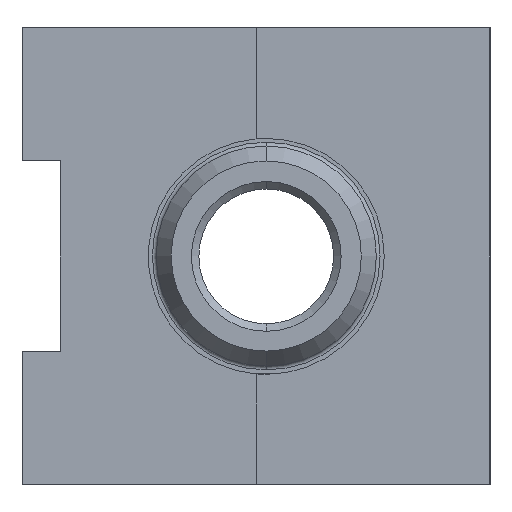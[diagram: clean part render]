
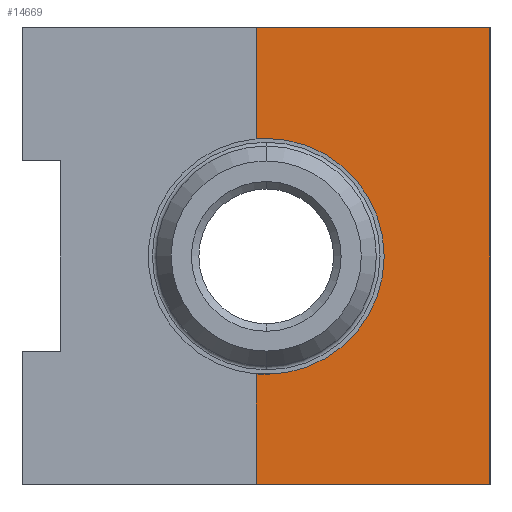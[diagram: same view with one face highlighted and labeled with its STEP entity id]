
A CAD part, left-side view. The second image highlights one B-rep face of the part: STEP entity #14669.
In plain terms, the highlighted face is planar.
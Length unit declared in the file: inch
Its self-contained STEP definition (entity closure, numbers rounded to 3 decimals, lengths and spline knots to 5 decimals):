
#445 = CARTESIAN_POINT ( 'NONE',  ( 1.2, -0.615, 0. ) ) ;
#660 = DIRECTION ( 'NONE',  ( 0., 1., 0. ) ) ;
#760 = DIRECTION ( 'NONE',  ( 1., 0., 0. ) ) ;
#808 = LINE ( 'NONE', #13899, #10339 ) ;
#1237 = VECTOR ( 'NONE', #19459, 39.37008 ) ;
#3102 = CARTESIAN_POINT ( 'NONE',  ( 0.29219, -0.615, 0. ) ) ;
#3241 = DIRECTION ( 'NONE',  ( 0., 0., -1. ) ) ;
#3429 = DIRECTION ( 'NONE',  ( 0., 0., -1. ) ) ;
#4312 = CARTESIAN_POINT ( 'NONE',  ( 0.29102, -0.6419, 0. ) ) ;
#4436 = CARTESIAN_POINT ( 'NONE',  ( 0., -0.615, 0. ) ) ;
#4488 = CARTESIAN_POINT ( 'NONE',  ( 0., 0., 0. ) ) ;
#4554 = CARTESIAN_POINT ( 'NONE',  ( 0., 0., 0. ) ) ;
#4571 = VERTEX_POINT ( 'NONE', #4436 ) ;
#4613 = ORIENTED_EDGE ( 'NONE', *, *, #21480, .F. ) ;
#4674 = DIRECTION ( 'NONE',  ( 0., 0., -1. ) ) ;
#4716 = EDGE_CURVE ( 'NONE', #19485, #11934, #10296, .T. ) ;
#5023 = ORIENTED_EDGE ( 'NONE', *, *, #16058, .F. ) ;
#5172 = EDGE_CURVE ( 'NONE', #4571, #15472, #20051, .T. ) ;
#5310 = ORIENTED_EDGE ( 'NONE', *, *, #5172, .T. ) ;
#5482 = EDGE_LOOP ( 'NONE', ( #20132, #5310, #8093, #5023, #17452, #15997, #4613, #18953 ) ) ;
#5793 = CARTESIAN_POINT ( 'NONE',  ( 1.2, 0., 0. ) ) ;
#6119 = PLANE ( 'NONE',  #20791 ) ;
#6831 = DIRECTION ( 'NONE',  ( -1., 0., 0. ) ) ;
#7147 = EDGE_CURVE ( 'NONE', #4571, #19485, #11410, .T. ) ;
#7215 = CARTESIAN_POINT ( 'NONE',  ( 0., -0.615, 0. ) ) ;
#7348 = EDGE_CURVE ( 'NONE', #7510, #20176, #13759, .T. ) ;
#7510 = VERTEX_POINT ( 'NONE', #19537 ) ;
#7834 = VECTOR ( 'NONE', #760, 39.37008 ) ;
#8061 = CARTESIAN_POINT ( 'NONE',  ( 0.60102, -0.6419, 0. ) ) ;
#8093 = ORIENTED_EDGE ( 'NONE', *, *, #18265, .F. ) ;
#8456 = DIRECTION ( 'NONE',  ( 1., 0., 0. ) ) ;
#8825 = AXIS2_PLACEMENT_3D ( 'NONE', #16921, #3429, #13758 ) ;
#9224 = CIRCLE ( 'NONE', #13730, 0.31 ) ;
#9228 = CARTESIAN_POINT ( 'NONE',  ( 1.2, -1.23, 0. ) ) ;
#9567 = VECTOR ( 'NONE', #660, 39.37008 ) ;
#9961 = AXIS2_PLACEMENT_3D ( 'NONE', #13256, #3241, #6831 ) ;
#10296 = LINE ( 'NONE', #11714, #15863 ) ;
#10339 = VECTOR ( 'NONE', #20507, 39.37008 ) ;
#11410 = LINE ( 'NONE', #4554, #1237 ) ;
#11714 = CARTESIAN_POINT ( 'NONE',  ( 0., -1.23, 0. ) ) ;
#11934 = VERTEX_POINT ( 'NONE', #9228 ) ;
#11993 = VERTEX_POINT ( 'NONE', #4312 ) ;
#12537 = DIRECTION ( 'NONE',  ( 0., 0., 1. ) ) ;
#12639 = DIRECTION ( 'NONE',  ( 1., 0., 0. ) ) ;
#12935 = EDGE_CURVE ( 'NONE', #7510, #18237, #808, .T. ) ;
#12994 = CIRCLE ( 'NONE', #8825, 0.31 ) ;
#13256 = CARTESIAN_POINT ( 'NONE',  ( 0.60102, -0.6419, 0. ) ) ;
#13730 = AXIS2_PLACEMENT_3D ( 'NONE', #8061, #4674, #16347 ) ;
#13758 = DIRECTION ( 'NONE',  ( -1., 0., 0. ) ) ;
#13759 = CIRCLE ( 'NONE', #9961, 0.31 ) ;
#13899 = CARTESIAN_POINT ( 'NONE',  ( 0., -0.615, 0. ) ) ;
#14614 = CARTESIAN_POINT ( 'NONE',  ( 0.91102, -0.6419, 0. ) ) ;
#14669 = ADVANCED_FACE ( 'NONE', ( #21001 ), #6119, .F. ) ;
#15472 = VERTEX_POINT ( 'NONE', #3102 ) ;
#15712 = LINE ( 'NONE', #5793, #9567 ) ;
#15863 = VECTOR ( 'NONE', #8456, 39.37008 ) ;
#15997 = ORIENTED_EDGE ( 'NONE', *, *, #12935, .T. ) ;
#16058 = EDGE_CURVE ( 'NONE', #20176, #11993, #9224, .T. ) ;
#16347 = DIRECTION ( 'NONE',  ( -1., 0., 0. ) ) ;
#16921 = CARTESIAN_POINT ( 'NONE',  ( 0.60102, -0.6419, 0. ) ) ;
#17452 = ORIENTED_EDGE ( 'NONE', *, *, #7348, .F. ) ;
#18237 = VERTEX_POINT ( 'NONE', #445 ) ;
#18265 = EDGE_CURVE ( 'NONE', #11993, #15472, #12994, .T. ) ;
#18590 = CARTESIAN_POINT ( 'NONE',  ( 0., -1.23, 0. ) ) ;
#18953 = ORIENTED_EDGE ( 'NONE', *, *, #4716, .F. ) ;
#19459 = DIRECTION ( 'NONE',  ( 0., -1., 0. ) ) ;
#19485 = VERTEX_POINT ( 'NONE', #18590 ) ;
#19537 = CARTESIAN_POINT ( 'NONE',  ( 0.90985, -0.615, 0. ) ) ;
#20051 = LINE ( 'NONE', #7215, #7834 ) ;
#20132 = ORIENTED_EDGE ( 'NONE', *, *, #7147, .F. ) ;
#20176 = VERTEX_POINT ( 'NONE', #14614 ) ;
#20507 = DIRECTION ( 'NONE',  ( 1., 0., 0. ) ) ;
#20791 = AXIS2_PLACEMENT_3D ( 'NONE', #4488, #12537, #12639 ) ;
#21001 = FACE_OUTER_BOUND ( 'NONE', #5482, .T. ) ;
#21480 = EDGE_CURVE ( 'NONE', #11934, #18237, #15712, .T. ) ;
